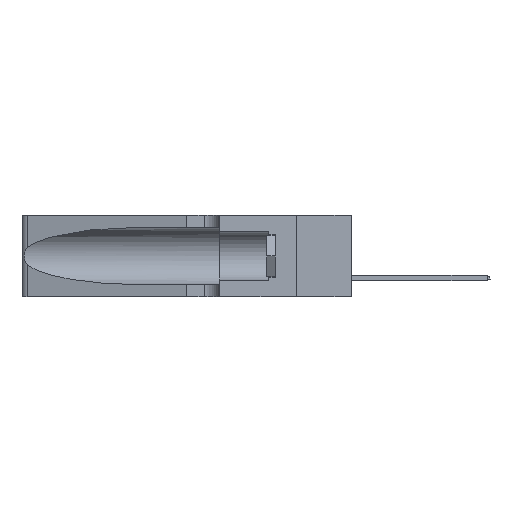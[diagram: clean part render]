
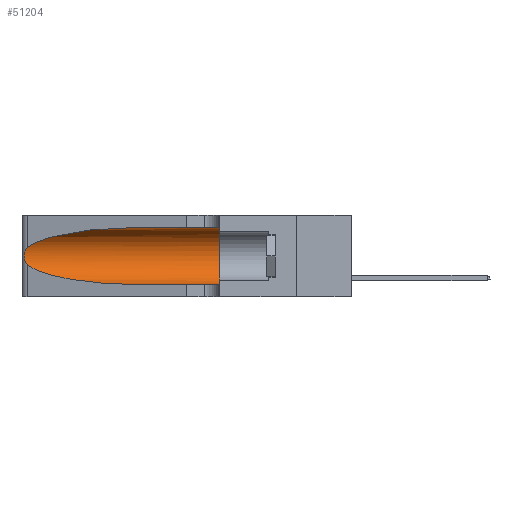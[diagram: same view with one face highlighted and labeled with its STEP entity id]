
A CAD part, left-side view. The second image highlights one B-rep face of the part: STEP entity #51204.
In plain terms, the highlighted cylindrical face has radius 3.308 mm (diameter 6.617 mm), a partial arc.
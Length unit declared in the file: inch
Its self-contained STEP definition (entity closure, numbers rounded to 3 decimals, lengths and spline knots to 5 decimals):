
#2109 = B_SPLINE_CURVE_WITH_KNOTS ( 'NONE', 3,
 ( #34369, #10925, #10248, #38456, #18823, #6673, #38634, #18659, #34708, #22878, #43232, #31008, #14299, #39156 ),
 .UNSPECIFIED., .F., .F.,
 ( 4, 2, 2, 2, 2, 2, 4 ),
 ( 0., 0.00027, 0.00053, 0.00107, 0.0016, 0.00187, 0.00214 ),
 .UNSPECIFIED. ) ;
#2233 = FACE_OUTER_BOUND ( 'NONE', #50202, .T. ) ;
#2499 = VERTEX_POINT ( 'NONE', #27845 ) ;
#2628 = DIRECTION ( 'NONE',  ( 0., 1., 0. ) ) ;
#2861 = ORIENTED_EDGE ( 'NONE', *, *, #12561, .T. ) ;
#3962 = CARTESIAN_POINT ( 'NONE',  ( 0.1305, 0.35, 0.31525 ) ) ;
#4305 = ORIENTED_EDGE ( 'NONE', *, *, #28157, .T. ) ;
#4621 = DIRECTION ( 'NONE',  ( 0., 0., -1. ) ) ;
#5967 = LINE ( 'NONE', #41181, #39459 ) ;
#6282 = CARTESIAN_POINT ( 'NONE',  ( 0.18966, 0.96281, 0.05475 ) ) ;
#6509 = CARTESIAN_POINT ( 'NONE',  ( 0.1305, 0.35, 0.185 ) ) ;
#6673 = CARTESIAN_POINT ( 'NONE',  ( 0.26018, 1.23835, 0.19895 ) ) ;
#9918 = CARTESIAN_POINT ( 'NONE',  ( 0.1305, 0.72297, 0.31525 ) ) ;
#10248 = CARTESIAN_POINT ( 'NONE',  ( 0.25639, 1.23184, 0.21858 ) ) ;
#10707 = CARTESIAN_POINT ( 'NONE',  ( 0.2373, 1.15595, 0.08982 ) ) ;
#10925 = CARTESIAN_POINT ( 'NONE',  ( 0.25555, 1.22994, 0.2215 ) ) ;
#12561 = EDGE_CURVE ( 'NONE', #14276, #26119, #43627, .T. ) ;
#13705 = CARTESIAN_POINT ( 'NONE',  ( 0.1305, 1.61858, 0.31525 ) ) ;
#14276 = VERTEX_POINT ( 'NONE', #9918 ) ;
#14299 = CARTESIAN_POINT ( 'NONE',  ( 0.25555, 1.22993, 0.14849 ) ) ;
#18659 = CARTESIAN_POINT ( 'NONE',  ( 0.26075, 1.23896, 0.178 ) ) ;
#18823 = CARTESIAN_POINT ( 'NONE',  ( 0.25854, 1.2359, 0.20912 ) ) ;
#19173 = CARTESIAN_POINT ( 'NONE',  ( 0.1305, 0.72297, 0.31525 ) ) ;
#20818 = VERTEX_POINT ( 'NONE', #3962 ) ;
#22878 = CARTESIAN_POINT ( 'NONE',  ( 0.25856, 1.23593, 0.16098 ) ) ;
#23142 = AXIS2_PLACEMENT_3D ( 'NONE', #6509, #2628, #39168 ) ;
#24378 = DIRECTION ( 'NONE',  ( 0., -1., 0. ) ) ;
#24709 = EDGE_CURVE ( 'NONE', #26119, #41833, #2109, .T. ) ;
#26119 = VERTEX_POINT ( 'NONE', #51505 ) ;
#26245 = VERTEX_POINT ( 'NONE', #52022 ) ;
#27845 = CARTESIAN_POINT ( 'NONE',  ( 0.1305, 0.72297, 0.05475 ) ) ;
#28157 = EDGE_CURVE ( 'NONE', #41833, #2499, #33184, .T. ) ;
#29457 = ORIENTED_EDGE ( 'NONE', *, *, #24709, .T. ) ;
#30485 = EDGE_CURVE ( 'NONE', #2499, #26245, #5967, .T. ) ;
#30615 = CARTESIAN_POINT ( 'NONE',  ( 0.1305, 0.72297, 0.05475 ) ) ;
#31008 = CARTESIAN_POINT ( 'NONE',  ( 0.25639, 1.23186, 0.15144 ) ) ;
#33184 =( BOUNDED_CURVE ( )  B_SPLINE_CURVE ( 3, ( #37693, #10707, #6282, #30615 ),
 .UNSPECIFIED., .F., .F. ) 
 B_SPLINE_CURVE_WITH_KNOTS ( ( 4, 4 ),
 ( 3.44316, 4.71239 ),
 .UNSPECIFIED. ) 
 CURVE ( )  GEOMETRIC_REPRESENTATION_ITEM ( )  RATIONAL_B_SPLINE_CURVE ( ( 1., 0.87, 0.87, 1. ) ) 
 REPRESENTATION_ITEM ( '' )  );
#34369 = CARTESIAN_POINT ( 'NONE',  ( 0.25487, 1.22718, 0.22369 ) ) ;
#34685 = ORIENTED_EDGE ( 'NONE', *, *, #30485, .T. ) ;
#34708 = CARTESIAN_POINT ( 'NONE',  ( 0.26017, 1.23833, 0.17102 ) ) ;
#35594 = CARTESIAN_POINT ( 'NONE',  ( 0.25487, 1.22718, 0.22369 ) ) ;
#37060 = ORIENTED_EDGE ( 'NONE', *, *, #37335, .F. ) ;
#37230 = VECTOR ( 'NONE', #37338, 39.37008 ) ;
#37335 = EDGE_CURVE ( 'NONE', #14276, #20818, #37845, .T. ) ;
#37338 = DIRECTION ( 'NONE',  ( 0., -1., 0. ) ) ;
#37439 = DIRECTION ( 'NONE',  ( 0., -1., 0. ) ) ;
#37693 = CARTESIAN_POINT ( 'NONE',  ( 0.25487, 1.22718, 0.14631 ) ) ;
#37845 = LINE ( 'NONE', #13705, #37230 ) ;
#38428 = ORIENTED_EDGE ( 'NONE', *, *, #45701, .F. ) ;
#38456 = CARTESIAN_POINT ( 'NONE',  ( 0.25787, 1.23484, 0.2124 ) ) ;
#38634 = CARTESIAN_POINT ( 'NONE',  ( 0.26075, 1.23896, 0.19203 ) ) ;
#38768 = CARTESIAN_POINT ( 'NONE',  ( 0.25487, 1.22718, 0.14631 ) ) ;
#39156 = CARTESIAN_POINT ( 'NONE',  ( 0.25487, 1.22718, 0.14631 ) ) ;
#39168 = DIRECTION ( 'NONE',  ( 0., 0., 1. ) ) ;
#39459 = VECTOR ( 'NONE', #37439, 39.37008 ) ;
#41005 = CARTESIAN_POINT ( 'NONE',  ( 0.1305, 1.61858, 0.185 ) ) ;
#41181 = CARTESIAN_POINT ( 'NONE',  ( 0.1305, 1.61858, 0.05475 ) ) ;
#41833 = VERTEX_POINT ( 'NONE', #38768 ) ;
#42305 = AXIS2_PLACEMENT_3D ( 'NONE', #41005, #24378, #4621 ) ;
#43232 = CARTESIAN_POINT ( 'NONE',  ( 0.25789, 1.23486, 0.15765 ) ) ;
#43238 = CARTESIAN_POINT ( 'NONE',  ( 0.18966, 0.96281, 0.31525 ) ) ;
#43627 =( BOUNDED_CURVE ( )  B_SPLINE_CURVE ( 3, ( #19173, #43238, #51296, #35594 ),
 .UNSPECIFIED., .F., .F. ) 
 B_SPLINE_CURVE_WITH_KNOTS ( ( 4, 4 ),
 ( 1.5708, 2.84003 ),
 .UNSPECIFIED. ) 
 CURVE ( )  GEOMETRIC_REPRESENTATION_ITEM ( )  RATIONAL_B_SPLINE_CURVE ( ( 1., 0.87, 0.87, 1. ) ) 
 REPRESENTATION_ITEM ( '' )  );
#44577 = CYLINDRICAL_SURFACE ( 'NONE', #42305, 0.13025 ) ;
#45701 = EDGE_CURVE ( 'NONE', #20818, #26245, #50296, .T. ) ;
#50202 = EDGE_LOOP ( 'NONE', ( #2861, #29457, #4305, #34685, #38428, #37060 ) ) ;
#50296 = CIRCLE ( 'NONE', #23142, 0.13025 ) ;
#51204 = ADVANCED_FACE ( 'NONE', ( #2233 ), #44577, .F. ) ;
#51296 = CARTESIAN_POINT ( 'NONE',  ( 0.2373, 1.15595, 0.28018 ) ) ;
#51505 = CARTESIAN_POINT ( 'NONE',  ( 0.25487, 1.22718, 0.22369 ) ) ;
#52022 = CARTESIAN_POINT ( 'NONE',  ( 0.1305, 0.35, 0.05475 ) ) ;
